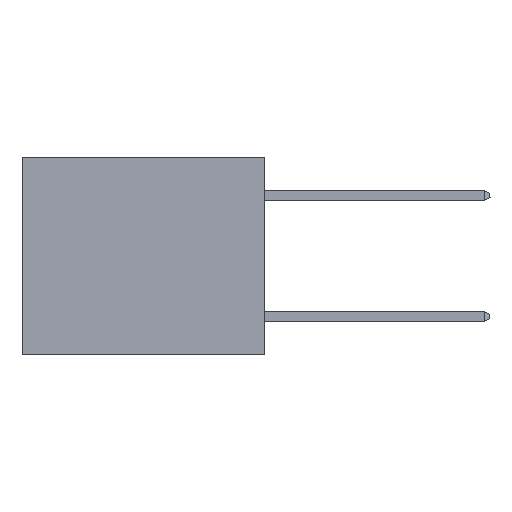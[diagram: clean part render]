
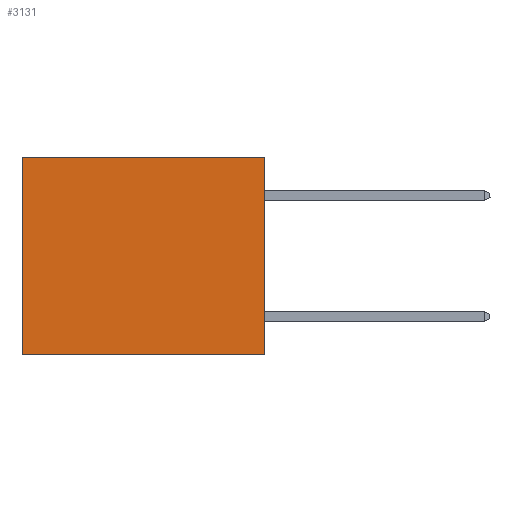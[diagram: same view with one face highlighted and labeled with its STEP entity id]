
A CAD part, left-side view. The second image highlights one B-rep face of the part: STEP entity #3131.
In plain terms, the highlighted planar face has unit normal (-1, 0, 0).
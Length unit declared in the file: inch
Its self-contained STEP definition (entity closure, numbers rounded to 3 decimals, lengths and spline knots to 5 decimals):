
#262 = CARTESIAN_POINT ( 'NONE',  ( 0.3165, 0.6, 0. ) ) ;
#726 = FACE_OUTER_BOUND ( 'NONE', #1572, .T. ) ;
#827 = CARTESIAN_POINT ( 'NONE',  ( 0.3165, 0., -0.49 ) ) ;
#1504 = LINE ( 'NONE', #10565, #7636 ) ;
#1572 = EDGE_LOOP ( 'NONE', ( #8365, #16549, #4832, #3386 ) ) ;
#1627 = EDGE_CURVE ( 'NONE', #15012, #10924, #23091, .T. ) ;
#2616 = LINE ( 'NONE', #9916, #24870 ) ;
#3131 = ADVANCED_FACE ( 'NONE', ( #726 ), #4916, .F. ) ;
#3386 = ORIENTED_EDGE ( 'NONE', *, *, #19037, .T. ) ;
#3411 = VERTEX_POINT ( 'NONE', #262 ) ;
#3572 = DIRECTION ( 'NONE',  ( 0., 0., -1. ) ) ;
#3819 = DIRECTION ( 'NONE',  ( 0., 1., 0. ) ) ;
#4661 = CARTESIAN_POINT ( 'NONE',  ( 0.3165, 0., -0.49 ) ) ;
#4832 = ORIENTED_EDGE ( 'NONE', *, *, #1627, .F. ) ;
#4916 = PLANE ( 'NONE',  #19886 ) ;
#6921 = DIRECTION ( 'NONE',  ( 1., 0., 0. ) ) ;
#7599 = CARTESIAN_POINT ( 'NONE',  ( 0.3165, 0., -0.49 ) ) ;
#7636 = VECTOR ( 'NONE', #20368, 39.37008 ) ;
#8365 = ORIENTED_EDGE ( 'NONE', *, *, #19854, .T. ) ;
#8684 = CARTESIAN_POINT ( 'NONE',  ( 0.3165, 0., 0. ) ) ;
#9916 = CARTESIAN_POINT ( 'NONE',  ( 0.3165, 0., 0. ) ) ;
#10565 = CARTESIAN_POINT ( 'NONE',  ( 0.3165, 0.6, -0.49 ) ) ;
#10924 = VERTEX_POINT ( 'NONE', #4661 ) ;
#11885 = DIRECTION ( 'NONE',  ( 0., 1., 0. ) ) ;
#15012 = VERTEX_POINT ( 'NONE', #8684 ) ;
#16549 = ORIENTED_EDGE ( 'NONE', *, *, #19191, .F. ) ;
#16777 = CARTESIAN_POINT ( 'NONE',  ( 0.3165, 0., -0.49 ) ) ;
#17960 = VECTOR ( 'NONE', #18445, 39.37008 ) ;
#18445 = DIRECTION ( 'NONE',  ( 0., 0., -1. ) ) ;
#19037 = EDGE_CURVE ( 'NONE', #15012, #3411, #2616, .T. ) ;
#19191 = EDGE_CURVE ( 'NONE', #10924, #21067, #20567, .T. ) ;
#19356 = VECTOR ( 'NONE', #3819, 39.37008 ) ;
#19854 = EDGE_CURVE ( 'NONE', #3411, #21067, #1504, .T. ) ;
#19886 = AXIS2_PLACEMENT_3D ( 'NONE', #16777, #6921, #3572 ) ;
#20101 = CARTESIAN_POINT ( 'NONE',  ( 0.3165, 0.6, -0.49 ) ) ;
#20368 = DIRECTION ( 'NONE',  ( 0., 0., -1. ) ) ;
#20567 = LINE ( 'NONE', #7599, #19356 ) ;
#21067 = VERTEX_POINT ( 'NONE', #20101 ) ;
#23091 = LINE ( 'NONE', #827, #17960 ) ;
#24870 = VECTOR ( 'NONE', #11885, 39.37008 ) ;
